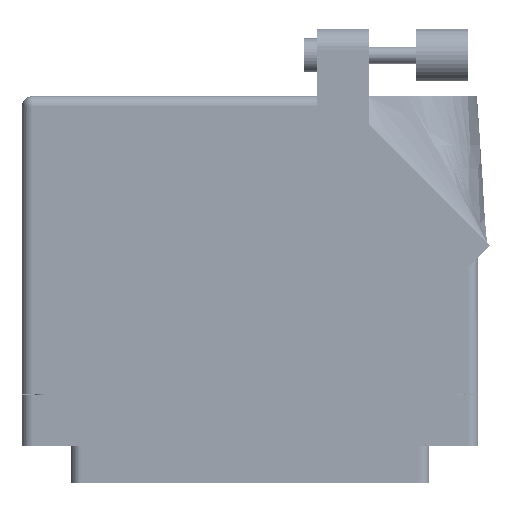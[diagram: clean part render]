
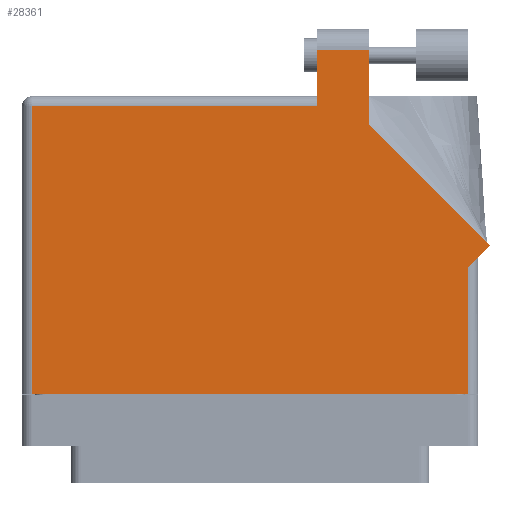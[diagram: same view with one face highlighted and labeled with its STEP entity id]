
A CAD part, front view. The second image highlights one B-rep face of the part: STEP entity #28361.
In plain terms, the highlighted face is planar.
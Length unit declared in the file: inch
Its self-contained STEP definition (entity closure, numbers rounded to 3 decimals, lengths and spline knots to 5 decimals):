
#1204 = DIRECTION ( 'NONE',  ( 0., 1., 0. ) ) ;
#2044 = DIRECTION ( 'NONE',  ( 0., 1., 0. ) ) ;
#2691 = ORIENTED_EDGE ( 'NONE', *, *, #14691, .T. ) ;
#3419 = DIRECTION ( 'NONE',  ( 0., -1., 0. ) ) ;
#3773 = DIRECTION ( 'NONE',  ( -1., 0., 0. ) ) ;
#5208 = VECTOR ( 'NONE', #1204, 39.37008 ) ;
#5577 = VECTOR ( 'NONE', #10630, 39.37008 ) ;
#7885 = CARTESIAN_POINT ( 'NONE',  ( 1.297, 0.653, 0.617 ) ) ;
#9109 = CARTESIAN_POINT ( 'NONE',  ( 0.399, 1.675, 0.617 ) ) ;
#9661 = DIRECTION ( 'NONE',  ( 0.707, 0.707, 0. ) ) ;
#9854 = EDGE_CURVE ( 'NONE', #65489, #39208, #68067, .T. ) ;
#10630 = DIRECTION ( 'NONE',  ( -0.707, 0.707, 0. ) ) ;
#13498 = EDGE_CURVE ( 'NONE', #66597, #46333, #39843, .T. ) ;
#14691 = EDGE_CURVE ( 'NONE', #39208, #48770, #57743, .T. ) ;
#15181 = VERTEX_POINT ( 'NONE', #29183 ) ;
#15892 = LINE ( 'NONE', #18728, #18552 ) ;
#16322 = DIRECTION ( 'NONE',  ( 0., -1., 0. ) ) ;
#16558 = DIRECTION ( 'NONE',  ( -1., 0., 0. ) ) ;
#17692 = EDGE_CURVE ( 'NONE', #65353, #40894, #48912, .T. ) ;
#17914 = CARTESIAN_POINT ( 'NONE',  ( -1.297, -0.1, 0.617 ) ) ;
#18552 = VECTOR ( 'NONE', #2044, 39.37008 ) ;
#18728 = CARTESIAN_POINT ( 'NONE',  ( 1.297, 0.715, 0.617 ) ) ;
#21160 = CARTESIAN_POINT ( 'NONE',  ( 0.399, 1.95, 0.617 ) ) ;
#22211 = VERTEX_POINT ( 'NONE', #52979 ) ;
#22480 = ORIENTED_EDGE ( 'NONE', *, *, #71205, .T. ) ;
#23816 = LINE ( 'NONE', #9109, #38090 ) ;
#24385 = ORIENTED_EDGE ( 'NONE', *, *, #13498, .T. ) ;
#27486 = VECTOR ( 'NONE', #67015, 39.37008 ) ;
#28361 = ADVANCED_FACE ( 'NONE', ( #53479 ), #71956, .F. ) ;
#28926 = EDGE_CURVE ( 'NONE', #15181, #66597, #15892, .T. ) ;
#29183 = CARTESIAN_POINT ( 'NONE',  ( 1.297, -0.1, 0.617 ) ) ;
#30189 = LINE ( 'NONE', #57595, #5208 ) ;
#33661 = ORIENTED_EDGE ( 'NONE', *, *, #67411, .T. ) ;
#37892 = DIRECTION ( 'NONE',  ( -1., 0., 0. ) ) ;
#37923 = CARTESIAN_POINT ( 'NONE',  ( -1.359, 1.675, 0.617 ) ) ;
#38090 = VECTOR ( 'NONE', #16322, 39.37008 ) ;
#38134 = CARTESIAN_POINT ( 'NONE',  ( 1.359, 0.715, 0.617 ) ) ;
#39101 = CARTESIAN_POINT ( 'NONE',  ( 1.42971, 0.78571, 0.617 ) ) ;
#39196 = CARTESIAN_POINT ( 'NONE',  ( 0.399, 1.95, 0.617 ) ) ;
#39208 = VERTEX_POINT ( 'NONE', #49284 ) ;
#39843 = LINE ( 'NONE', #38134, #48725 ) ;
#40150 = ORIENTED_EDGE ( 'NONE', *, *, #17692, .T. ) ;
#40894 = VERTEX_POINT ( 'NONE', #39196 ) ;
#42125 = VECTOR ( 'NONE', #16558, 39.37008 ) ;
#42316 = CARTESIAN_POINT ( 'NONE',  ( -1.297, -0.1, 0.617 ) ) ;
#43955 = AXIS2_PLACEMENT_3D ( 'NONE', #37923, #49135, #3773 ) ;
#44478 = CARTESIAN_POINT ( 'NONE',  ( -1.359, 1.613, 0.617 ) ) ;
#44654 = ORIENTED_EDGE ( 'NONE', *, *, #59923, .T. ) ;
#46333 = VERTEX_POINT ( 'NONE', #70799 ) ;
#47143 = VECTOR ( 'NONE', #37892, 39.37008 ) ;
#48725 = VECTOR ( 'NONE', #9661, 39.37008 ) ;
#48770 = VERTEX_POINT ( 'NONE', #17914 ) ;
#48912 = LINE ( 'NONE', #21160, #47143 ) ;
#49135 = DIRECTION ( 'NONE',  ( 0., 0., -1. ) ) ;
#49284 = CARTESIAN_POINT ( 'NONE',  ( -1.297, 1.613, 0.617 ) ) ;
#50495 = CARTESIAN_POINT ( 'NONE',  ( -1.359, -0.1, 0.617 ) ) ;
#51457 = LINE ( 'NONE', #50495, #27486 ) ;
#52979 = CARTESIAN_POINT ( 'NONE',  ( 0.706, 1.50942, 0.617 ) ) ;
#53479 = FACE_OUTER_BOUND ( 'NONE', #60513, .T. ) ;
#53593 = ORIENTED_EDGE ( 'NONE', *, *, #59566, .T. ) ;
#55175 = ORIENTED_EDGE ( 'NONE', *, *, #28926, .T. ) ;
#57595 = CARTESIAN_POINT ( 'NONE',  ( 0.706, 1.50942, 0.617 ) ) ;
#57743 = LINE ( 'NONE', #42316, #64030 ) ;
#59566 = EDGE_CURVE ( 'NONE', #22211, #65353, #30189, .T. ) ;
#59923 = EDGE_CURVE ( 'NONE', #48770, #15181, #51457, .T. ) ;
#60418 = ORIENTED_EDGE ( 'NONE', *, *, #9854, .T. ) ;
#60513 = EDGE_LOOP ( 'NONE', ( #53593, #40150, #33661, #60418, #2691, #44654, #55175, #24385, #22480 ) ) ;
#62032 = CARTESIAN_POINT ( 'NONE',  ( 0.399, 1.613, 0.617 ) ) ;
#64030 = VECTOR ( 'NONE', #3419, 39.37008 ) ;
#65353 = VERTEX_POINT ( 'NONE', #72109 ) ;
#65395 = LINE ( 'NONE', #39101, #5577 ) ;
#65489 = VERTEX_POINT ( 'NONE', #62032 ) ;
#66597 = VERTEX_POINT ( 'NONE', #7885 ) ;
#67015 = DIRECTION ( 'NONE',  ( 1., 0., 0. ) ) ;
#67411 = EDGE_CURVE ( 'NONE', #40894, #65489, #23816, .T. ) ;
#68067 = LINE ( 'NONE', #44478, #42125 ) ;
#70799 = CARTESIAN_POINT ( 'NONE',  ( 1.42971, 0.78571, 0.617 ) ) ;
#71205 = EDGE_CURVE ( 'NONE', #46333, #22211, #65395, .T. ) ;
#71956 = PLANE ( 'NONE',  #43955 ) ;
#72109 = CARTESIAN_POINT ( 'NONE',  ( 0.706, 1.95, 0.617 ) ) ;
